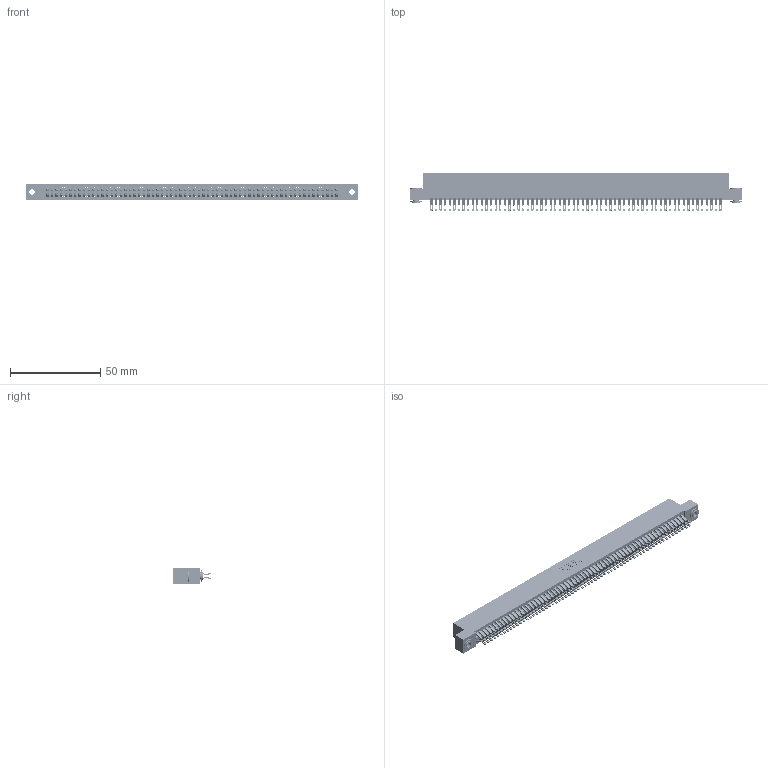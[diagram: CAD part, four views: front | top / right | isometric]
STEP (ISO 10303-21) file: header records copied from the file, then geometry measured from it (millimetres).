
FILE_DESCRIPTION (( 'STEP AP203' ), '1' );
FILE_NAME ('395-128-555-203.STEP', '2018-12-04T12:36:53', ( '' ), ( '' ), 'SwSTEP 2.0', 'SolidWorks 2016', '' );
FILE_SCHEMA (( 'CONFIG_CONTROL_DESIGN' ));
Length unit declared in the file: inch
Products named in the file (4): 395-128-555-203; 345 Part_Flush Mounting Lugs - 0.156 Dia-TH; 345-292-001_555 Tail; 345-250-002_345-250-002-102
Assembly tree (131 placements, depth 2):
  395-128-555-203
    345 Part_Flush Mounting Lugs - 0.156 Dia-TH
    345-292-001_555 Tail  x128
    345-250-002_345-250-002-102  x2
Bounding box: 183.77 x 21.13 x 9.4 mm (x, y, z)
Volume: 18446.4 mm3; surface area: 29189.2 mm2
Topology: 131 solids, 131 shells, 7332 faces, 23073 edges, 15378 vertices
Faces by surface type: plane 4058, cylinder 3266, cone 8
Entity records: 48230 total; most frequent: CARTESIAN_POINT 8073, ORIENTED_EDGE 7970, DIRECTION 7091, EDGE_CURVE 3985, LINE 3553, VECTOR 3553, VERTEX_POINT 2654, AXIS2_PLACEMENT_3D 1769
